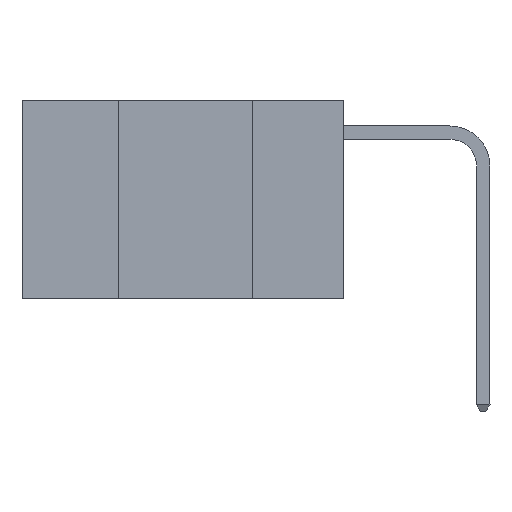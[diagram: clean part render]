
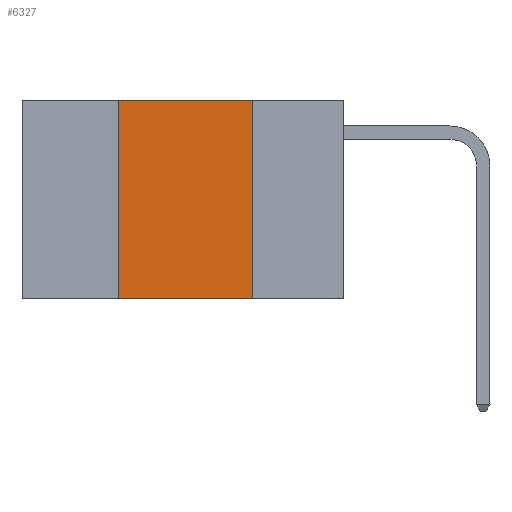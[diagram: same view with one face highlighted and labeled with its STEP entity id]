
A CAD part, left-side view. The second image highlights one B-rep face of the part: STEP entity #6327.
In plain terms, the highlighted planar face has unit normal (-1, 0, 0).
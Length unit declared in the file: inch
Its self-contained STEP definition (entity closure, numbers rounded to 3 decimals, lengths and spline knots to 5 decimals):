
#2159 = VERTEX_POINT ( 'NONE', #7860 ) ;
#2513 = CARTESIAN_POINT ( 'NONE',  ( 0., 0.6, 0. ) ) ;
#2877 = EDGE_LOOP ( 'NONE', ( #7316, #6105, #4006, #7269 ) ) ;
#3341 = VECTOR ( 'NONE', #12630, 39.37008 ) ;
#3359 = VECTOR ( 'NONE', #6374, 39.37008 ) ;
#3392 = CARTESIAN_POINT ( 'NONE',  ( 0., 0.6, 0. ) ) ;
#3561 = PLANE ( 'NONE',  #8898 ) ;
#4006 = ORIENTED_EDGE ( 'NONE', *, *, #9371, .F. ) ;
#4106 = CARTESIAN_POINT ( 'NONE',  ( 0., 0.6, -0.37 ) ) ;
#4709 = CARTESIAN_POINT ( 'NONE',  ( 0., 0.42, 0. ) ) ;
#4841 = VERTEX_POINT ( 'NONE', #6596 ) ;
#5125 = DIRECTION ( 'NONE',  ( 0., -1., 0. ) ) ;
#5446 = CARTESIAN_POINT ( 'NONE',  ( 0., 0.42, 0. ) ) ;
#5610 = DIRECTION ( 'NONE',  ( 1., 0., 0. ) ) ;
#5831 = VERTEX_POINT ( 'NONE', #9800 ) ;
#6105 = ORIENTED_EDGE ( 'NONE', *, *, #12051, .F. ) ;
#6327 = ADVANCED_FACE ( 'NONE', ( #11374 ), #3561, .F. ) ;
#6350 = VECTOR ( 'NONE', #10075, 39.37008 ) ;
#6374 = DIRECTION ( 'NONE',  ( 0., 0., 1. ) ) ;
#6596 = CARTESIAN_POINT ( 'NONE',  ( 0., 0.17, -0.37 ) ) ;
#7269 = ORIENTED_EDGE ( 'NONE', *, *, #12391, .T. ) ;
#7316 = ORIENTED_EDGE ( 'NONE', *, *, #9119, .F. ) ;
#7860 = CARTESIAN_POINT ( 'NONE',  ( 0., 0.42, -0.37 ) ) ;
#8329 = LINE ( 'NONE', #10711, #3341 ) ;
#8731 = LINE ( 'NONE', #4106, #10621 ) ;
#8857 = LINE ( 'NONE', #3392, #6350 ) ;
#8898 = AXIS2_PLACEMENT_3D ( 'NONE', #2513, #5610, #12178 ) ;
#9119 = EDGE_CURVE ( 'NONE', #5831, #4841, #8329, .T. ) ;
#9371 = EDGE_CURVE ( 'NONE', #2159, #10295, #11219, .T. ) ;
#9800 = CARTESIAN_POINT ( 'NONE',  ( 0., 0.17, 0. ) ) ;
#10075 = DIRECTION ( 'NONE',  ( 0., -1., 0. ) ) ;
#10295 = VERTEX_POINT ( 'NONE', #4709 ) ;
#10621 = VECTOR ( 'NONE', #5125, 39.37008 ) ;
#10711 = CARTESIAN_POINT ( 'NONE',  ( 0., 0.17, 0. ) ) ;
#11219 = LINE ( 'NONE', #5446, #3359 ) ;
#11374 = FACE_OUTER_BOUND ( 'NONE', #2877, .T. ) ;
#12051 = EDGE_CURVE ( 'NONE', #10295, #5831, #8857, .T. ) ;
#12178 = DIRECTION ( 'NONE',  ( 0., 0., -1. ) ) ;
#12391 = EDGE_CURVE ( 'NONE', #2159, #4841, #8731, .T. ) ;
#12630 = DIRECTION ( 'NONE',  ( 0., 0., -1. ) ) ;
